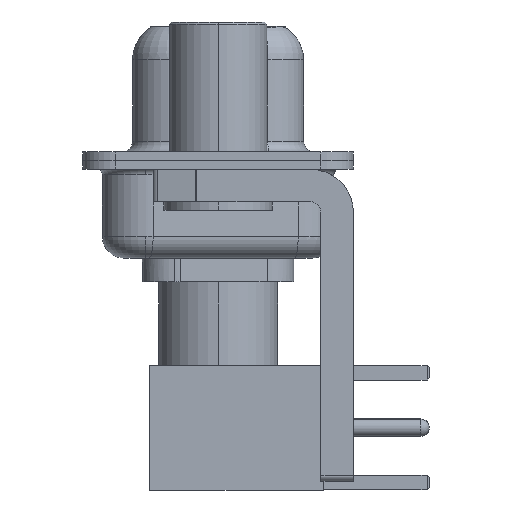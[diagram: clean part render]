
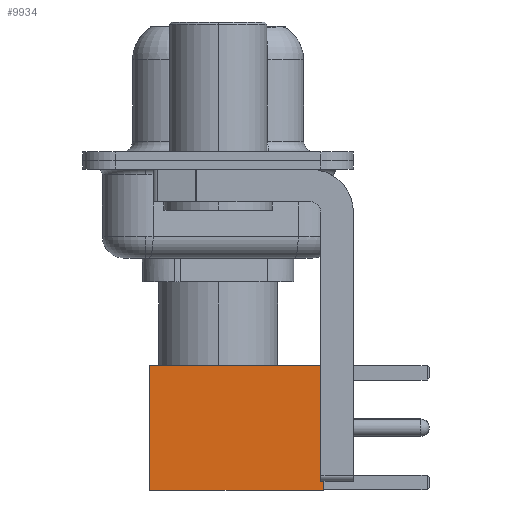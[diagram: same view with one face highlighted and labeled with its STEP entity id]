
A CAD part, left-side view. The second image highlights one B-rep face of the part: STEP entity #9934.
In plain terms, the highlighted face is planar.
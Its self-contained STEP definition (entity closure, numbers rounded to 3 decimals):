
#1036 = ORIENTED_EDGE ( 'NONE', *, *, #5152, .T. ) ;
#1103 = VECTOR ( 'NONE', #14309, 1000. ) ;
#1585 = CARTESIAN_POINT ( 'NONE',  ( -2.875, 2.875, 0. ) ) ;
#2358 = CARTESIAN_POINT ( 'NONE',  ( 0., 2.875, 0. ) ) ;
#2481 = VECTOR ( 'NONE', #14705, 1000. ) ;
#2643 = VERTEX_POINT ( 'NONE', #7036 ) ;
#3915 = VERTEX_POINT ( 'NONE', #1585 ) ;
#4154 = VECTOR ( 'NONE', #12897, 1000. ) ;
#4249 = AXIS2_PLACEMENT_3D ( 'NONE', #10880, #20570, #15240 ) ;
#5152 = EDGE_CURVE ( 'NONE', #19955, #3915, #8816, .T. ) ;
#5588 = PLANE ( 'NONE',  #4249 ) ;
#5702 = FACE_OUTER_BOUND ( 'NONE', #7690, .T. ) ;
#5847 = DIRECTION ( 'NONE',  ( -1., 0., 0. ) ) ;
#7036 = CARTESIAN_POINT ( 'NONE',  ( 2.875, 2.875, 8. ) ) ;
#7690 = EDGE_LOOP ( 'NONE', ( #12520, #1036, #15976, #18631 ) ) ;
#8816 = LINE ( 'NONE', #2358, #12434 ) ;
#9307 = LINE ( 'NONE', #19076, #4154 ) ;
#9632 = LINE ( 'NONE', #17694, #1103 ) ;
#9934 = ADVANCED_FACE ( 'NONE', ( #5702 ), #5588, .T. ) ;
#10260 = CARTESIAN_POINT ( 'NONE',  ( -2.875, 2.875, 8. ) ) ;
#10880 = CARTESIAN_POINT ( 'NONE',  ( 2.875, 2.875, 0. ) ) ;
#12434 = VECTOR ( 'NONE', #5847, 1000. ) ;
#12520 = ORIENTED_EDGE ( 'NONE', *, *, #15831, .T. ) ;
#12897 = DIRECTION ( 'NONE',  ( 0., 0., -1. ) ) ;
#14309 = DIRECTION ( 'NONE',  ( -1., 0., 0. ) ) ;
#14705 = DIRECTION ( 'NONE',  ( 0., 0., -1. ) ) ;
#15048 = EDGE_CURVE ( 'NONE', #2643, #15423, #9632, .T. ) ;
#15240 = DIRECTION ( 'NONE',  ( 0., 0., 1. ) ) ;
#15423 = VERTEX_POINT ( 'NONE', #10260 ) ;
#15551 = EDGE_CURVE ( 'NONE', #15423, #3915, #9307, .T. ) ;
#15831 = EDGE_CURVE ( 'NONE', #2643, #19955, #17890, .T. ) ;
#15976 = ORIENTED_EDGE ( 'NONE', *, *, #15551, .F. ) ;
#16404 = CARTESIAN_POINT ( 'NONE',  ( 2.875, 2.875, 0. ) ) ;
#16846 = CARTESIAN_POINT ( 'NONE',  ( 2.875, 2.875, 0. ) ) ;
#17694 = CARTESIAN_POINT ( 'NONE',  ( 0., 2.875, 8. ) ) ;
#17890 = LINE ( 'NONE', #16404, #2481 ) ;
#18631 = ORIENTED_EDGE ( 'NONE', *, *, #15048, .F. ) ;
#19076 = CARTESIAN_POINT ( 'NONE',  ( -2.875, 2.875, 0. ) ) ;
#19955 = VERTEX_POINT ( 'NONE', #16846 ) ;
#20570 = DIRECTION ( 'NONE',  ( 0., 1., 0. ) ) ;
